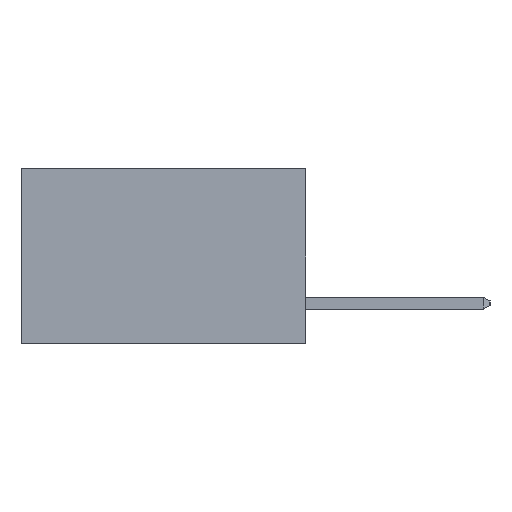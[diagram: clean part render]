
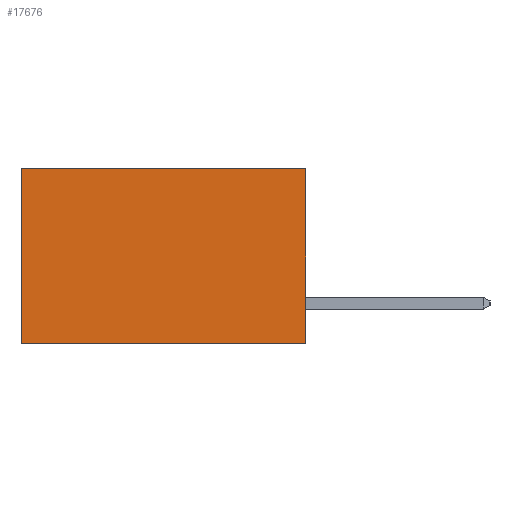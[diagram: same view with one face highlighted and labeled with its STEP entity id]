
A CAD part, left-side view. The second image highlights one B-rep face of the part: STEP entity #17676.
In plain terms, the highlighted planar face has unit normal (-1, 0, 0).
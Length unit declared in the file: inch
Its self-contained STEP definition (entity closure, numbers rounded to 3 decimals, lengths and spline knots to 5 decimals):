
#28 = VERTEX_POINT ( 'NONE', #15958 ) ;
#491 = VECTOR ( 'NONE', #4535, 39.37008 ) ;
#629 = EDGE_CURVE ( 'NONE', #28, #3323, #4105, .T. ) ;
#1674 = CARTESIAN_POINT ( 'NONE',  ( 0.2615, 0.6, -0.37 ) ) ;
#3323 = VERTEX_POINT ( 'NONE', #1674 ) ;
#4105 = LINE ( 'NONE', #4599, #491 ) ;
#4535 = DIRECTION ( 'NONE',  ( 0., 1., 0. ) ) ;
#4599 = CARTESIAN_POINT ( 'NONE',  ( 0.2615, 0., -0.37 ) ) ;
#4624 = VECTOR ( 'NONE', #7233, 39.37008 ) ;
#4706 = DIRECTION ( 'NONE',  ( 0., 0., -1. ) ) ;
#4999 = EDGE_CURVE ( 'NONE', #12663, #3323, #15814, .T. ) ;
#5416 = CARTESIAN_POINT ( 'NONE',  ( 0.2615, 0., 0. ) ) ;
#5596 = CARTESIAN_POINT ( 'NONE',  ( 0.2615, 0., -0.37 ) ) ;
#6358 = CARTESIAN_POINT ( 'NONE',  ( 0.2615, 0.6, -0.37 ) ) ;
#6714 = ORIENTED_EDGE ( 'NONE', *, *, #629, .F. ) ;
#6768 = ORIENTED_EDGE ( 'NONE', *, *, #4999, .T. ) ;
#7151 = VECTOR ( 'NONE', #8926, 39.37008 ) ;
#7169 = DIRECTION ( 'NONE',  ( 0., 0., -1. ) ) ;
#7233 = DIRECTION ( 'NONE',  ( 0., 0., -1. ) ) ;
#8501 = FACE_OUTER_BOUND ( 'NONE', #16885, .T. ) ;
#8651 = EDGE_CURVE ( 'NONE', #13133, #12663, #19520, .T. ) ;
#8926 = DIRECTION ( 'NONE',  ( 0., 1., 0. ) ) ;
#9464 = CARTESIAN_POINT ( 'NONE',  ( 0.2615, 0., 0. ) ) ;
#10301 = CARTESIAN_POINT ( 'NONE',  ( 0.2615, 0., -0.37 ) ) ;
#10621 = ORIENTED_EDGE ( 'NONE', *, *, #8651, .T. ) ;
#11680 = VECTOR ( 'NONE', #4706, 39.37008 ) ;
#12663 = VERTEX_POINT ( 'NONE', #15030 ) ;
#13133 = VERTEX_POINT ( 'NONE', #5416 ) ;
#14990 = PLANE ( 'NONE',  #15544 ) ;
#15030 = CARTESIAN_POINT ( 'NONE',  ( 0.2615, 0.6, 0. ) ) ;
#15544 = AXIS2_PLACEMENT_3D ( 'NONE', #10301, #16560, #7169 ) ;
#15814 = LINE ( 'NONE', #6358, #11680 ) ;
#15820 = ORIENTED_EDGE ( 'NONE', *, *, #15836, .F. ) ;
#15836 = EDGE_CURVE ( 'NONE', #13133, #28, #16678, .T. ) ;
#15958 = CARTESIAN_POINT ( 'NONE',  ( 0.2615, 0., -0.37 ) ) ;
#16560 = DIRECTION ( 'NONE',  ( 1., 0., 0. ) ) ;
#16678 = LINE ( 'NONE', #5596, #4624 ) ;
#16885 = EDGE_LOOP ( 'NONE', ( #6768, #6714, #15820, #10621 ) ) ;
#17676 = ADVANCED_FACE ( 'NONE', ( #8501 ), #14990, .F. ) ;
#19520 = LINE ( 'NONE', #9464, #7151 ) ;
